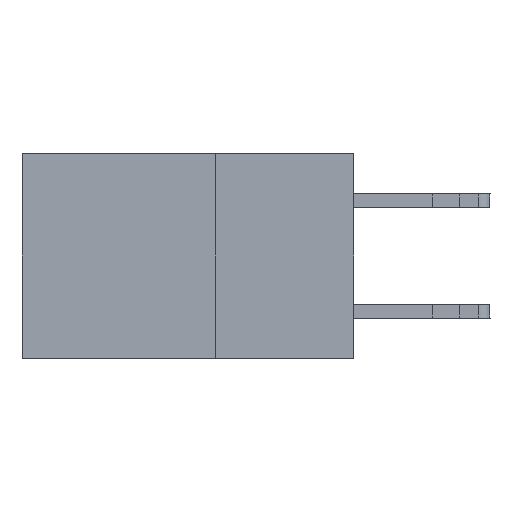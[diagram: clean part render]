
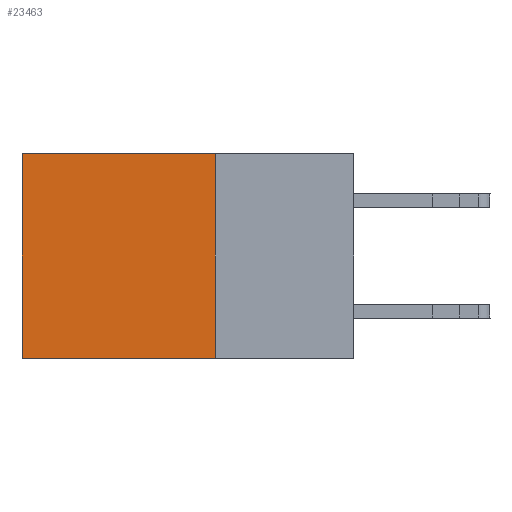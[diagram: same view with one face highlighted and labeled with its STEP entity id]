
A CAD part, left-side view. The second image highlights one B-rep face of the part: STEP entity #23463.
In plain terms, the highlighted planar face has unit normal (-1, 0, 0).
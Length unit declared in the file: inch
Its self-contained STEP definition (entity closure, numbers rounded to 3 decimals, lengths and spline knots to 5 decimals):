
#471 = LINE ( 'NONE', #9548, #12305 ) ;
#1135 = LINE ( 'NONE', #36768, #30051 ) ;
#3216 = ORIENTED_EDGE ( 'NONE', *, *, #26936, .F. ) ;
#4998 = CARTESIAN_POINT ( 'NONE',  ( 0.2875, 0.6, 0. ) ) ;
#5096 = FACE_OUTER_BOUND ( 'NONE', #32276, .T. ) ;
#7203 = PLANE ( 'NONE',  #11036 ) ;
#7283 = CARTESIAN_POINT ( 'NONE',  ( 0.2875, 0.25, -0.37 ) ) ;
#7660 = EDGE_CURVE ( 'NONE', #26035, #31912, #23519, .T. ) ;
#7965 = DIRECTION ( 'NONE',  ( 0., 0., -1. ) ) ;
#8587 = ORIENTED_EDGE ( 'NONE', *, *, #29134, .F. ) ;
#8651 = VECTOR ( 'NONE', #34709, 39.37008 ) ;
#9548 = CARTESIAN_POINT ( 'NONE',  ( 0.2875, 0.25, -0.37 ) ) ;
#11036 = AXIS2_PLACEMENT_3D ( 'NONE', #30338, #35732, #24323 ) ;
#11607 = CARTESIAN_POINT ( 'NONE',  ( 0.2875, 0.6, -0.37 ) ) ;
#12205 = DIRECTION ( 'NONE',  ( 0., 1., 0. ) ) ;
#12305 = VECTOR ( 'NONE', #12205, 39.37008 ) ;
#12471 = CARTESIAN_POINT ( 'NONE',  ( 0.2875, 0.25, 0. ) ) ;
#12832 = ORIENTED_EDGE ( 'NONE', *, *, #15850, .T. ) ;
#13739 = ORIENTED_EDGE ( 'NONE', *, *, #7660, .T. ) ;
#14411 = DIRECTION ( 'NONE',  ( 0., 1., 0. ) ) ;
#15850 = EDGE_CURVE ( 'NONE', #32085, #26035, #28358, .T. ) ;
#20061 = CARTESIAN_POINT ( 'NONE',  ( 0.2875, 0.25, 0. ) ) ;
#20396 = VERTEX_POINT ( 'NONE', #7283 ) ;
#23463 = ADVANCED_FACE ( 'NONE', ( #5096 ), #7203, .F. ) ;
#23519 = LINE ( 'NONE', #28988, #8651 ) ;
#24323 = DIRECTION ( 'NONE',  ( 0., 0., -1. ) ) ;
#26035 = VERTEX_POINT ( 'NONE', #4998 ) ;
#26936 = EDGE_CURVE ( 'NONE', #32085, #20396, #1135, .T. ) ;
#28358 = LINE ( 'NONE', #20061, #35521 ) ;
#28988 = CARTESIAN_POINT ( 'NONE',  ( 0.2875, 0.6, 0. ) ) ;
#29134 = EDGE_CURVE ( 'NONE', #20396, #31912, #471, .T. ) ;
#30051 = VECTOR ( 'NONE', #7965, 39.37008 ) ;
#30338 = CARTESIAN_POINT ( 'NONE',  ( 0.2875, 0.25, 0. ) ) ;
#31912 = VERTEX_POINT ( 'NONE', #11607 ) ;
#32085 = VERTEX_POINT ( 'NONE', #12471 ) ;
#32276 = EDGE_LOOP ( 'NONE', ( #13739, #8587, #3216, #12832 ) ) ;
#34709 = DIRECTION ( 'NONE',  ( 0., 0., -1. ) ) ;
#35521 = VECTOR ( 'NONE', #14411, 39.37008 ) ;
#35732 = DIRECTION ( 'NONE',  ( 1., 0., 0. ) ) ;
#36768 = CARTESIAN_POINT ( 'NONE',  ( 0.2875, 0.25, 0. ) ) ;
